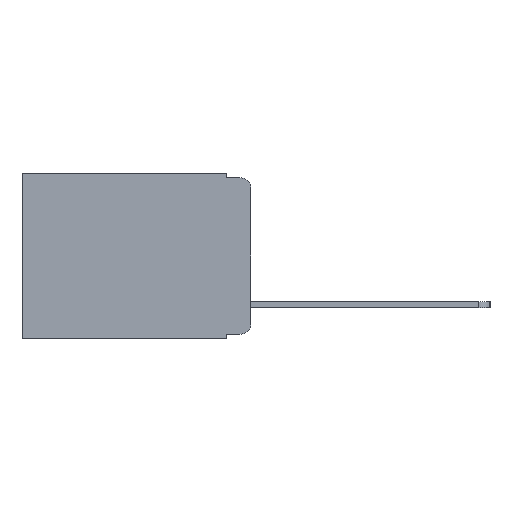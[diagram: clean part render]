
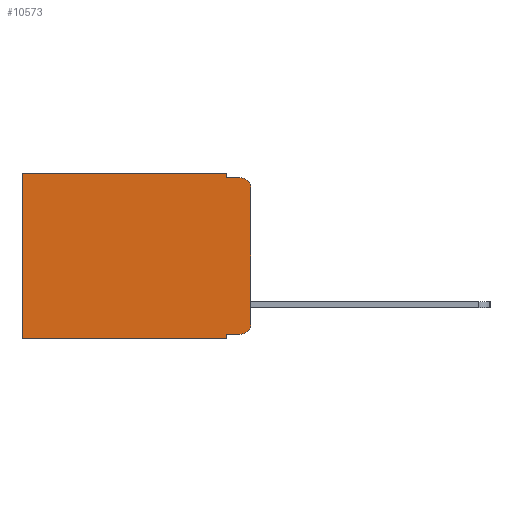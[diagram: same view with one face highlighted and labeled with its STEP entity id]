
A CAD part, left-side view. The second image highlights one B-rep face of the part: STEP entity #10573.
In plain terms, the highlighted planar face has unit normal (-1, 0, 0).
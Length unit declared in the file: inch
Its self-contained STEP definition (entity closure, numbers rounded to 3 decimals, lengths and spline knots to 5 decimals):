
#54 = VERTEX_POINT ( 'NONE', #7787 ) ;
#135 = EDGE_CURVE ( 'NONE', #11229, #5046, #455, .T. ) ;
#322 = VECTOR ( 'NONE', #3111, 39.37008 ) ;
#330 = LINE ( 'NONE', #11236, #6010 ) ;
#337 = VERTEX_POINT ( 'NONE', #7625 ) ;
#455 = LINE ( 'NONE', #4269, #322 ) ;
#523 = VECTOR ( 'NONE', #4286, 39.37008 ) ;
#694 = LINE ( 'NONE', #1585, #11779 ) ;
#889 = ORIENTED_EDGE ( 'NONE', *, *, #2867, .F. ) ;
#1040 = DIRECTION ( 'NONE',  ( 0., 0., -1. ) ) ;
#1080 = ORIENTED_EDGE ( 'NONE', *, *, #2966, .F. ) ;
#1083 = LINE ( 'NONE', #11117, #10967 ) ;
#1167 = ORIENTED_EDGE ( 'NONE', *, *, #7199, .T. ) ;
#1256 = VERTEX_POINT ( 'NONE', #11105 ) ;
#1283 = CIRCLE ( 'NONE', #10038, 0.02 ) ;
#1307 = ORIENTED_EDGE ( 'NONE', *, *, #3017, .T. ) ;
#1410 = ORIENTED_EDGE ( 'NONE', *, *, #135, .F. ) ;
#1492 = DIRECTION ( 'NONE',  ( 0., -1., 0. ) ) ;
#1504 = ORIENTED_EDGE ( 'NONE', *, *, #3040, .F. ) ;
#1585 = CARTESIAN_POINT ( 'NONE',  ( 0.298, 0.051, -0.333 ) ) ;
#1690 = ORIENTED_EDGE ( 'NONE', *, *, #3059, .T. ) ;
#1753 = DIRECTION ( 'NONE',  ( 0., 0., -1. ) ) ;
#1842 = LINE ( 'NONE', #5376, #9415 ) ;
#1889 = ORIENTED_EDGE ( 'NONE', *, *, #3148, .T. ) ;
#2715 = EDGE_CURVE ( 'NONE', #7670, #1256, #6022, .T. ) ;
#2824 = EDGE_CURVE ( 'NONE', #7670, #54, #1283, .T. ) ;
#2867 = EDGE_CURVE ( 'NONE', #3526, #54, #5885, .T. ) ;
#2891 = CARTESIAN_POINT ( 'NONE',  ( 0.298, 0., -0.03 ) ) ;
#2966 = EDGE_CURVE ( 'NONE', #4902, #3526, #1842, .T. ) ;
#2980 = CARTESIAN_POINT ( 'NONE',  ( 0.298, 0.02, -0.313 ) ) ;
#3017 = EDGE_CURVE ( 'NONE', #337, #5046, #1083, .T. ) ;
#3040 = EDGE_CURVE ( 'NONE', #4838, #11229, #330, .T. ) ;
#3059 = EDGE_CURVE ( 'NONE', #4838, #6772, #694, .T. ) ;
#3111 = DIRECTION ( 'NONE',  ( 0., 1., 0. ) ) ;
#3148 = EDGE_CURVE ( 'NONE', #6772, #1256, #11335, .T. ) ;
#3319 = FACE_OUTER_BOUND ( 'NONE', #6649, .T. ) ;
#3526 = VERTEX_POINT ( 'NONE', #3748 ) ;
#3748 = CARTESIAN_POINT ( 'NONE',  ( 0.298, 0.051, -0.01 ) ) ;
#4269 = CARTESIAN_POINT ( 'NONE',  ( 0.298, 0., -0.343 ) ) ;
#4286 = DIRECTION ( 'NONE',  ( 0., -1., 0. ) ) ;
#4382 = CARTESIAN_POINT ( 'NONE',  ( 0.298, 0.473, -0.343 ) ) ;
#4533 = DIRECTION ( 'NONE',  ( -1., 0., 0. ) ) ;
#4682 = CARTESIAN_POINT ( 'NONE',  ( 0.298, 0.02, -0.333 ) ) ;
#4838 = VERTEX_POINT ( 'NONE', #7653 ) ;
#4902 = VERTEX_POINT ( 'NONE', #5412 ) ;
#5046 = VERTEX_POINT ( 'NONE', #4382 ) ;
#5261 = DIRECTION ( 'NONE',  ( 0., 0., -1. ) ) ;
#5376 = CARTESIAN_POINT ( 'NONE',  ( 0.298, 0.051, 0. ) ) ;
#5412 = CARTESIAN_POINT ( 'NONE',  ( 0.298, 0.051, 0. ) ) ;
#5885 = LINE ( 'NONE', #6327, #523 ) ;
#6010 = VECTOR ( 'NONE', #11226, 39.37008 ) ;
#6022 = LINE ( 'NONE', #11347, #10729 ) ;
#6138 = AXIS2_PLACEMENT_3D ( 'NONE', #7034, #6978, #6926 ) ;
#6263 = AXIS2_PLACEMENT_3D ( 'NONE', #2980, #11189, #11180 ) ;
#6327 = CARTESIAN_POINT ( 'NONE',  ( 0.298, 0.051, -0.01 ) ) ;
#6649 = EDGE_LOOP ( 'NONE', ( #8505, #10314, #889, #1080, #1167, #1307, #1410, #1504, #1690, #1889 ) ) ;
#6772 = VERTEX_POINT ( 'NONE', #4682 ) ;
#6926 = DIRECTION ( 'NONE',  ( 0., 0., -1. ) ) ;
#6978 = DIRECTION ( 'NONE',  ( 1., 0., 0. ) ) ;
#7034 = CARTESIAN_POINT ( 'NONE',  ( 0.298, 0., 0. ) ) ;
#7177 = DIRECTION ( 'NONE',  ( 0., 1., 0. ) ) ;
#7199 = EDGE_CURVE ( 'NONE', #4902, #337, #9837, .T. ) ;
#7249 = CARTESIAN_POINT ( 'NONE',  ( 0.298, 0.02, -0.03 ) ) ;
#7625 = CARTESIAN_POINT ( 'NONE',  ( 0.298, 0.473, 0. ) ) ;
#7653 = CARTESIAN_POINT ( 'NONE',  ( 0.298, 0.051, -0.333 ) ) ;
#7670 = VERTEX_POINT ( 'NONE', #2891 ) ;
#7730 = CARTESIAN_POINT ( 'NONE',  ( 0.298, 0., 0. ) ) ;
#7787 = CARTESIAN_POINT ( 'NONE',  ( 0.298, 0.02, -0.01 ) ) ;
#7970 = DIRECTION ( 'NONE',  ( 0., 0., -1. ) ) ;
#8505 = ORIENTED_EDGE ( 'NONE', *, *, #2715, .F. ) ;
#8818 = CARTESIAN_POINT ( 'NONE',  ( 0.298, 0.051, -0.343 ) ) ;
#9415 = VECTOR ( 'NONE', #1753, 39.37008 ) ;
#9837 = LINE ( 'NONE', #7730, #11608 ) ;
#10038 = AXIS2_PLACEMENT_3D ( 'NONE', #7249, #4533, #5261 ) ;
#10314 = ORIENTED_EDGE ( 'NONE', *, *, #2824, .T. ) ;
#10573 = ADVANCED_FACE ( 'NONE', ( #3319 ), #11792, .F. ) ;
#10729 = VECTOR ( 'NONE', #7970, 39.37008 ) ;
#10967 = VECTOR ( 'NONE', #1040, 39.37008 ) ;
#11105 = CARTESIAN_POINT ( 'NONE',  ( 0.298, 0., -0.313 ) ) ;
#11117 = CARTESIAN_POINT ( 'NONE',  ( 0.298, 0.473, 0. ) ) ;
#11180 = DIRECTION ( 'NONE',  ( 0., 0., -1. ) ) ;
#11189 = DIRECTION ( 'NONE',  ( -1., 0., 0. ) ) ;
#11226 = DIRECTION ( 'NONE',  ( 0., 0., -1. ) ) ;
#11229 = VERTEX_POINT ( 'NONE', #8818 ) ;
#11236 = CARTESIAN_POINT ( 'NONE',  ( 0.298, 0.051, 0. ) ) ;
#11335 = CIRCLE ( 'NONE', #6263, 0.02 ) ;
#11347 = CARTESIAN_POINT ( 'NONE',  ( 0.298, 0., 0. ) ) ;
#11608 = VECTOR ( 'NONE', #7177, 39.37008 ) ;
#11779 = VECTOR ( 'NONE', #1492, 39.37008 ) ;
#11792 = PLANE ( 'NONE',  #6138 ) ;
